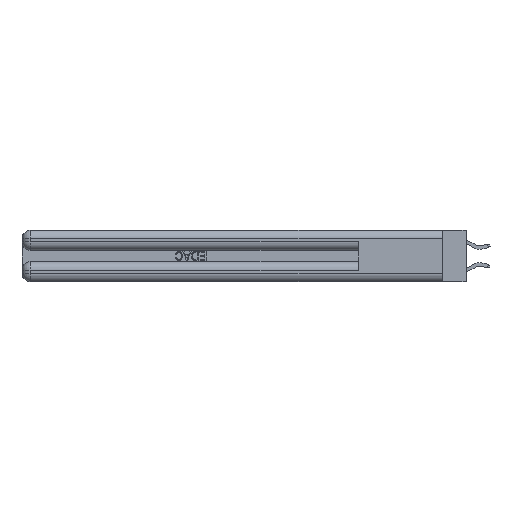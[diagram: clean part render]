
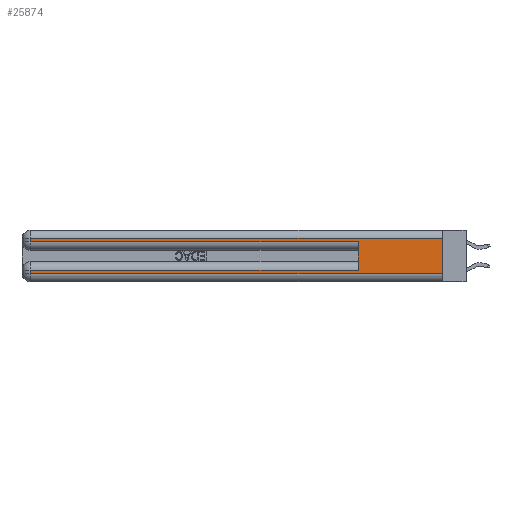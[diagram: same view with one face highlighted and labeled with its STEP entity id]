
A CAD part, left-side view. The second image highlights one B-rep face of the part: STEP entity #25874.
In plain terms, the highlighted planar face has unit normal (-1, 0, 0).
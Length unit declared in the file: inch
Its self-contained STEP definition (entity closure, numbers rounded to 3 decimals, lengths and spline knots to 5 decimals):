
#182 = CARTESIAN_POINT ( 'NONE',  ( 0., 0., 0.085 ) ) ;
#261 = CARTESIAN_POINT ( 'NONE',  ( 0., 2.94, 0.06 ) ) ;
#559 = ORIENTED_EDGE ( 'NONE', *, *, #11337, .T. ) ;
#1620 = ORIENTED_EDGE ( 'NONE', *, *, #10990, .T. ) ;
#2180 = LINE ( 'NONE', #25102, #6719 ) ;
#2252 = ORIENTED_EDGE ( 'NONE', *, *, #13290, .T. ) ;
#2856 = DIRECTION ( 'NONE',  ( 0., -1., 0. ) ) ;
#2945 = DIRECTION ( 'NONE',  ( 0., 0., -1. ) ) ;
#4130 = ORIENTED_EDGE ( 'NONE', *, *, #22945, .F. ) ;
#4292 = EDGE_CURVE ( 'NONE', #20604, #11643, #24232, .T. ) ;
#4679 = VERTEX_POINT ( 'NONE', #261 ) ;
#4805 = ORIENTED_EDGE ( 'NONE', *, *, #7040, .F. ) ;
#4947 = VECTOR ( 'NONE', #25152, 39.37008 ) ;
#5672 = VECTOR ( 'NONE', #26963, 39.37008 ) ;
#6371 = LINE ( 'NONE', #18265, #5672 ) ;
#6719 = VECTOR ( 'NONE', #27289, 39.37008 ) ;
#7040 = EDGE_CURVE ( 'NONE', #9145, #12589, #10902, .T. ) ;
#7254 = CARTESIAN_POINT ( 'NONE',  ( 0., 0., 0.37 ) ) ;
#7442 = CARTESIAN_POINT ( 'NONE',  ( 0., 2.94, 0.31 ) ) ;
#7828 = FACE_OUTER_BOUND ( 'NONE', #28765, .T. ) ;
#7845 = VECTOR ( 'NONE', #26899, 39.37008 ) ;
#8912 = CARTESIAN_POINT ( 'NONE',  ( 0., 0., 0.31 ) ) ;
#9145 = VERTEX_POINT ( 'NONE', #8912 ) ;
#10247 = CARTESIAN_POINT ( 'NONE',  ( 0., 2.94, 0.37 ) ) ;
#10289 = CARTESIAN_POINT ( 'NONE',  ( 0., 2.94, 0.085 ) ) ;
#10902 = LINE ( 'NONE', #7254, #4947 ) ;
#10990 = EDGE_CURVE ( 'NONE', #20759, #4679, #16328, .T. ) ;
#11093 = ORIENTED_EDGE ( 'NONE', *, *, #15174, .T. ) ;
#11337 = EDGE_CURVE ( 'NONE', #15010, #20759, #26342, .T. ) ;
#11643 = VERTEX_POINT ( 'NONE', #23521 ) ;
#12589 = VERTEX_POINT ( 'NONE', #24740 ) ;
#13290 = EDGE_CURVE ( 'NONE', #9145, #20604, #2180, .T. ) ;
#13935 = DIRECTION ( 'NONE',  ( 0., 0., -1. ) ) ;
#14056 = CARTESIAN_POINT ( 'NONE',  ( 0., 0., 0.06 ) ) ;
#14137 = CARTESIAN_POINT ( 'NONE',  ( 0., 0., 0.37 ) ) ;
#14685 = LINE ( 'NONE', #24794, #19900 ) ;
#15010 = VERTEX_POINT ( 'NONE', #26857 ) ;
#15174 = EDGE_CURVE ( 'NONE', #4679, #12589, #21524, .T. ) ;
#16328 = LINE ( 'NONE', #27217, #28049 ) ;
#16402 = DIRECTION ( 'NONE',  ( 1., 0., 0. ) ) ;
#18265 = CARTESIAN_POINT ( 'NONE',  ( 0., 0., 0.285 ) ) ;
#19900 = VECTOR ( 'NONE', #20437, 39.37008 ) ;
#20437 = DIRECTION ( 'NONE',  ( 0., 0., 1. ) ) ;
#20479 = EDGE_CURVE ( 'NONE', #11643, #23479, #6371, .T. ) ;
#20604 = VERTEX_POINT ( 'NONE', #7442 ) ;
#20759 = VERTEX_POINT ( 'NONE', #10289 ) ;
#20841 = VECTOR ( 'NONE', #2856, 39.37008 ) ;
#21524 = LINE ( 'NONE', #14056, #20841 ) ;
#22421 = CARTESIAN_POINT ( 'NONE',  ( 0., 0.6, 0.285 ) ) ;
#22945 = EDGE_CURVE ( 'NONE', #15010, #23479, #14685, .T. ) ;
#23404 = AXIS2_PLACEMENT_3D ( 'NONE', #14137, #16402, #2945 ) ;
#23479 = VERTEX_POINT ( 'NONE', #22421 ) ;
#23521 = CARTESIAN_POINT ( 'NONE',  ( 0., 2.94, 0.285 ) ) ;
#23549 = VECTOR ( 'NONE', #28023, 39.37008 ) ;
#24232 = LINE ( 'NONE', #10247, #23549 ) ;
#24678 = ORIENTED_EDGE ( 'NONE', *, *, #20479, .T. ) ;
#24740 = CARTESIAN_POINT ( 'NONE',  ( 0., 0., 0.06 ) ) ;
#24794 = CARTESIAN_POINT ( 'NONE',  ( 0., 0.6, 0.145 ) ) ;
#25102 = CARTESIAN_POINT ( 'NONE',  ( 0., 0., 0.31 ) ) ;
#25152 = DIRECTION ( 'NONE',  ( 0., 0., -1. ) ) ;
#25874 = ADVANCED_FACE ( 'NONE', ( #7828 ), #27410, .F. ) ;
#26342 = LINE ( 'NONE', #182, #7845 ) ;
#26768 = ORIENTED_EDGE ( 'NONE', *, *, #4292, .T. ) ;
#26857 = CARTESIAN_POINT ( 'NONE',  ( 0., 0.6, 0.085 ) ) ;
#26899 = DIRECTION ( 'NONE',  ( 0., 1., 0. ) ) ;
#26963 = DIRECTION ( 'NONE',  ( 0., -1., 0. ) ) ;
#27217 = CARTESIAN_POINT ( 'NONE',  ( 0., 2.94, 0.37 ) ) ;
#27289 = DIRECTION ( 'NONE',  ( 0., 1., 0. ) ) ;
#27410 = PLANE ( 'NONE',  #23404 ) ;
#28023 = DIRECTION ( 'NONE',  ( 0., 0., -1. ) ) ;
#28049 = VECTOR ( 'NONE', #13935, 39.37008 ) ;
#28765 = EDGE_LOOP ( 'NONE', ( #4805, #2252, #26768, #24678, #4130, #559, #1620, #11093 ) ) ;
